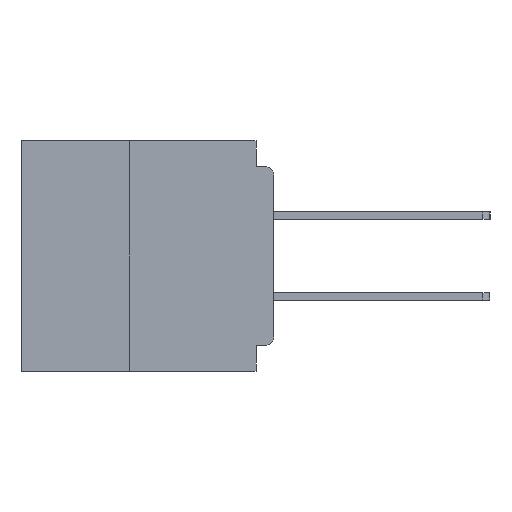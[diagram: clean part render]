
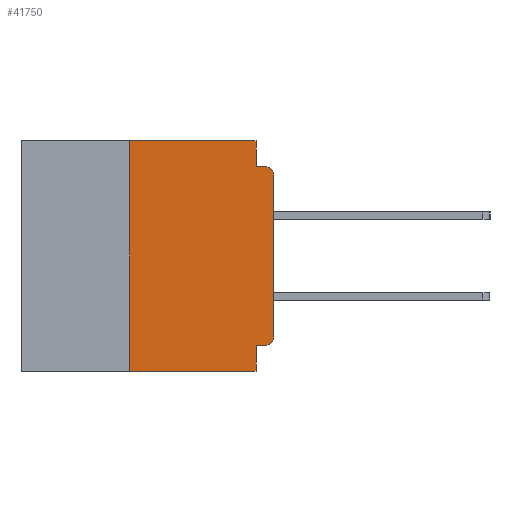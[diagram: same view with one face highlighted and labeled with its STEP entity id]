
A CAD part, left-side view. The second image highlights one B-rep face of the part: STEP entity #41750.
In plain terms, the highlighted planar face has unit normal (-1, 0, 0).
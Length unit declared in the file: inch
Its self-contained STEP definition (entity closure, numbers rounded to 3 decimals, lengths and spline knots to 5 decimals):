
#533 = CARTESIAN_POINT ( 'NONE',  ( 0., 0.031, -0.4 ) ) ;
#2035 = LINE ( 'NONE', #24218, #28513 ) ;
#2246 = CARTESIAN_POINT ( 'NONE',  ( 0., 0.031, -0.4 ) ) ;
#4105 = CARTESIAN_POINT ( 'NONE',  ( 0., 0., -0.06 ) ) ;
#4618 = ORIENTED_EDGE ( 'NONE', *, *, #30637, .T. ) ;
#5981 = DIRECTION ( 'NONE',  ( -1., 0., 0. ) ) ;
#6909 = DIRECTION ( 'NONE',  ( 0., 1., 0. ) ) ;
#7230 = VECTOR ( 'NONE', #14801, 39.37008 ) ;
#8299 = LINE ( 'NONE', #11329, #7230 ) ;
#9120 = DIRECTION ( 'NONE',  ( 0., 0., -1. ) ) ;
#9561 = ORIENTED_EDGE ( 'NONE', *, *, #21062, .T. ) ;
#9936 = DIRECTION ( 'NONE',  ( 0., -1., 0. ) ) ;
#10682 = CARTESIAN_POINT ( 'NONE',  ( 0., 0.015, -0.355 ) ) ;
#11329 = CARTESIAN_POINT ( 'NONE',  ( 0., 0.437, -0.4 ) ) ;
#11376 = ORIENTED_EDGE ( 'NONE', *, *, #38034, .F. ) ;
#11889 = VERTEX_POINT ( 'NONE', #10682 ) ;
#12315 = LINE ( 'NONE', #22651, #30592 ) ;
#13302 = CARTESIAN_POINT ( 'NONE',  ( 0., 0.25, -0.4 ) ) ;
#13506 = ORIENTED_EDGE ( 'NONE', *, *, #21529, .F. ) ;
#13833 = AXIS2_PLACEMENT_3D ( 'NONE', #26637, #5981, #30054 ) ;
#13979 = ORIENTED_EDGE ( 'NONE', *, *, #17918, .F. ) ;
#14801 = DIRECTION ( 'NONE',  ( 0., -1., 0. ) ) ;
#14829 = CIRCLE ( 'NONE', #13833, 0.015 ) ;
#15011 = VECTOR ( 'NONE', #6909, 39.37008 ) ;
#15554 = PLANE ( 'NONE',  #42016 ) ;
#15648 = VECTOR ( 'NONE', #9120, 39.37008 ) ;
#16190 = ORIENTED_EDGE ( 'NONE', *, *, #43481, .T. ) ;
#16653 = CARTESIAN_POINT ( 'NONE',  ( 0., 0.015, -0.34 ) ) ;
#17189 = CARTESIAN_POINT ( 'NONE',  ( 0., 0., -0.355 ) ) ;
#17255 = DIRECTION ( 'NONE',  ( 0., 0., -1. ) ) ;
#17918 = EDGE_CURVE ( 'NONE', #30643, #44458, #42886, .T. ) ;
#18732 = FACE_OUTER_BOUND ( 'NONE', #33224, .T. ) ;
#19205 = LINE ( 'NONE', #27118, #25146 ) ;
#19662 = VECTOR ( 'NONE', #24623, 39.37008 ) ;
#20128 = DIRECTION ( 'NONE',  ( 0., 0., -1. ) ) ;
#20139 = CARTESIAN_POINT ( 'NONE',  ( 0., 0.25, -0.4 ) ) ;
#20369 = EDGE_CURVE ( 'NONE', #21548, #35637, #19205, .T. ) ;
#21062 = EDGE_CURVE ( 'NONE', #38048, #44458, #8299, .T. ) ;
#21170 = CARTESIAN_POINT ( 'NONE',  ( 0., 0., 0. ) ) ;
#21529 = EDGE_CURVE ( 'NONE', #11889, #30643, #24216, .T. ) ;
#21548 = VERTEX_POINT ( 'NONE', #34412 ) ;
#22277 = CARTESIAN_POINT ( 'NONE',  ( 0., 0.015, -0.045 ) ) ;
#22525 = DIRECTION ( 'NONE',  ( 0., 0., -1. ) ) ;
#22543 = ORIENTED_EDGE ( 'NONE', *, *, #27064, .T. ) ;
#22651 = CARTESIAN_POINT ( 'NONE',  ( 0., 0., -0.045 ) ) ;
#24216 = LINE ( 'NONE', #17189, #15011 ) ;
#24218 = CARTESIAN_POINT ( 'NONE',  ( 0., 0.031, 0. ) ) ;
#24368 = AXIS2_PLACEMENT_3D ( 'NONE', #16653, #40503, #20128 ) ;
#24623 = DIRECTION ( 'NONE',  ( 0., 0., 1. ) ) ;
#24805 = CARTESIAN_POINT ( 'NONE',  ( 0., 0., -0.34 ) ) ;
#24894 = CARTESIAN_POINT ( 'NONE',  ( 0., 0.031, -0.045 ) ) ;
#25146 = VECTOR ( 'NONE', #9936, 39.37008 ) ;
#26637 = CARTESIAN_POINT ( 'NONE',  ( 0., 0.015, -0.06 ) ) ;
#27064 = EDGE_CURVE ( 'NONE', #29239, #32294, #14829, .T. ) ;
#27118 = CARTESIAN_POINT ( 'NONE',  ( 0., 0.437, 0. ) ) ;
#27879 = ORIENTED_EDGE ( 'NONE', *, *, #20369, .F. ) ;
#28239 = LINE ( 'NONE', #20139, #36186 ) ;
#28513 = VECTOR ( 'NONE', #17255, 39.37008 ) ;
#29239 = VERTEX_POINT ( 'NONE', #4105 ) ;
#29718 = ORIENTED_EDGE ( 'NONE', *, *, #41014, .F. ) ;
#30054 = DIRECTION ( 'NONE',  ( 0., 0., -1. ) ) ;
#30270 = CARTESIAN_POINT ( 'NONE',  ( 0., 0.031, -0.355 ) ) ;
#30592 = VECTOR ( 'NONE', #42985, 39.37008 ) ;
#30637 = EDGE_CURVE ( 'NONE', #11889, #38360, #35940, .T. ) ;
#30643 = VERTEX_POINT ( 'NONE', #30270 ) ;
#32294 = VERTEX_POINT ( 'NONE', #22277 ) ;
#33224 = EDGE_LOOP ( 'NONE', ( #16190, #22543, #29718, #42668, #27879, #11376, #9561, #13979, #13506, #4618 ) ) ;
#34317 = EDGE_CURVE ( 'NONE', #35637, #37024, #2035, .T. ) ;
#34412 = CARTESIAN_POINT ( 'NONE',  ( 0., 0.25, 0. ) ) ;
#35637 = VERTEX_POINT ( 'NONE', #37151 ) ;
#35940 = CIRCLE ( 'NONE', #24368, 0.015 ) ;
#36186 = VECTOR ( 'NONE', #40672, 39.37008 ) ;
#37024 = VERTEX_POINT ( 'NONE', #24894 ) ;
#37151 = CARTESIAN_POINT ( 'NONE',  ( 0., 0.031, 0. ) ) ;
#38034 = EDGE_CURVE ( 'NONE', #38048, #21548, #28239, .T. ) ;
#38048 = VERTEX_POINT ( 'NONE', #13302 ) ;
#38360 = VERTEX_POINT ( 'NONE', #24805 ) ;
#39404 = CARTESIAN_POINT ( 'NONE',  ( 0., 0.437, 0. ) ) ;
#40503 = DIRECTION ( 'NONE',  ( -1., 0., 0. ) ) ;
#40672 = DIRECTION ( 'NONE',  ( 0., 0., 1. ) ) ;
#41014 = EDGE_CURVE ( 'NONE', #37024, #32294, #12315, .T. ) ;
#41750 = ADVANCED_FACE ( 'NONE', ( #18732 ), #15554, .F. ) ;
#42016 = AXIS2_PLACEMENT_3D ( 'NONE', #39404, #42866, #22525 ) ;
#42668 = ORIENTED_EDGE ( 'NONE', *, *, #34317, .F. ) ;
#42866 = DIRECTION ( 'NONE',  ( 1., 0., 0. ) ) ;
#42886 = LINE ( 'NONE', #2246, #15648 ) ;
#42985 = DIRECTION ( 'NONE',  ( 0., -1., 0. ) ) ;
#43109 = LINE ( 'NONE', #21170, #19662 ) ;
#43481 = EDGE_CURVE ( 'NONE', #38360, #29239, #43109, .T. ) ;
#44458 = VERTEX_POINT ( 'NONE', #533 ) ;
